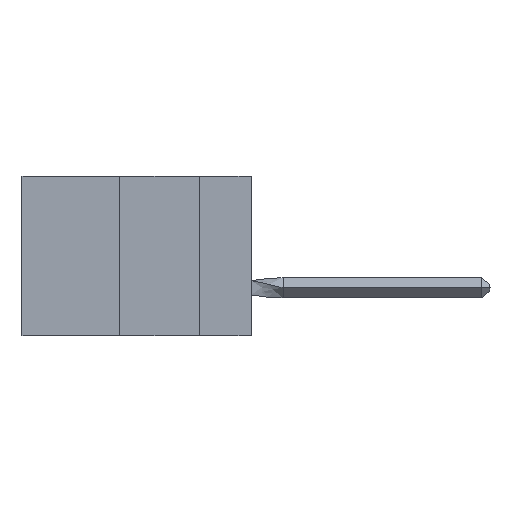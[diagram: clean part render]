
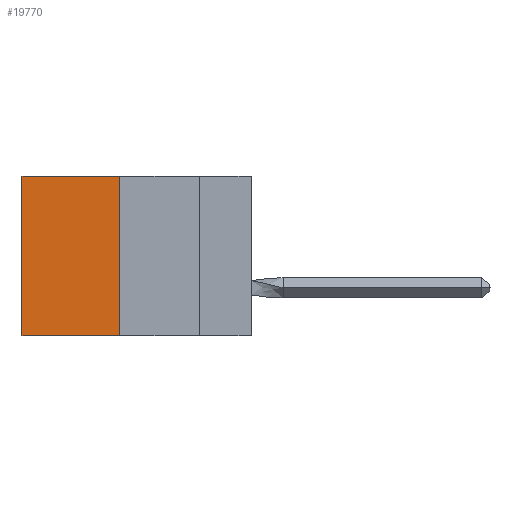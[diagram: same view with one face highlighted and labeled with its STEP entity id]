
A CAD part, left-side view. The second image highlights one B-rep face of the part: STEP entity #19770.
In plain terms, the highlighted planar face has unit normal (-1, 0, 0).
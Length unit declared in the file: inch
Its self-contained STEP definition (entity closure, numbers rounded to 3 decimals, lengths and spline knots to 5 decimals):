
#2408 = VERTEX_POINT ( 'NONE', #26722 ) ;
#3050 = VERTEX_POINT ( 'NONE', #18640 ) ;
#5060 = LINE ( 'NONE', #7306, #8090 ) ;
#5773 = DIRECTION ( 'NONE',  ( 1., 0., 0. ) ) ;
#5916 = CARTESIAN_POINT ( 'NONE',  ( 0.305, 0.413, -0.5 ) ) ;
#7297 = EDGE_CURVE ( 'NONE', #29053, #15346, #5060, .T. ) ;
#7306 = CARTESIAN_POINT ( 'NONE',  ( 0.305, 0.413, -0.5 ) ) ;
#8090 = VECTOR ( 'NONE', #20172, 39.37008 ) ;
#12396 = CARTESIAN_POINT ( 'NONE',  ( 0.305, 0.413, -0.5 ) ) ;
#14778 = VECTOR ( 'NONE', #28162, 39.37008 ) ;
#15084 = VECTOR ( 'NONE', #22329, 39.37008 ) ;
#15346 = VERTEX_POINT ( 'NONE', #33138 ) ;
#16229 = ORIENTED_EDGE ( 'NONE', *, *, #22057, .T. ) ;
#16317 = LINE ( 'NONE', #31427, #14778 ) ;
#16789 = EDGE_CURVE ( 'NONE', #3050, #15346, #28140, .T. ) ;
#17355 = LINE ( 'NONE', #12396, #22442 ) ;
#17820 = CARTESIAN_POINT ( 'NONE',  ( 0.305, 0.72, -0.5 ) ) ;
#18640 = CARTESIAN_POINT ( 'NONE',  ( 0.305, 0.72, 0. ) ) ;
#19770 = ADVANCED_FACE ( 'NONE', ( #37947 ), #38411, .F. ) ;
#19824 = EDGE_CURVE ( 'NONE', #2408, #29053, #17355, .T. ) ;
#20172 = DIRECTION ( 'NONE',  ( 0., 1., 0. ) ) ;
#22057 = EDGE_CURVE ( 'NONE', #2408, #3050, #16317, .T. ) ;
#22329 = DIRECTION ( 'NONE',  ( 0., 0., -1. ) ) ;
#22442 = VECTOR ( 'NONE', #28450, 39.37008 ) ;
#26722 = CARTESIAN_POINT ( 'NONE',  ( 0.305, 0.413, 0. ) ) ;
#28017 = AXIS2_PLACEMENT_3D ( 'NONE', #5916, #5773, #31833 ) ;
#28140 = LINE ( 'NONE', #17820, #15084 ) ;
#28162 = DIRECTION ( 'NONE',  ( 0., 1., 0. ) ) ;
#28173 = ORIENTED_EDGE ( 'NONE', *, *, #7297, .F. ) ;
#28450 = DIRECTION ( 'NONE',  ( 0., 0., -1. ) ) ;
#29053 = VERTEX_POINT ( 'NONE', #39777 ) ;
#31427 = CARTESIAN_POINT ( 'NONE',  ( 0.305, 0.413, 0. ) ) ;
#31610 = ORIENTED_EDGE ( 'NONE', *, *, #16789, .T. ) ;
#31833 = DIRECTION ( 'NONE',  ( 0., 0., -1. ) ) ;
#33138 = CARTESIAN_POINT ( 'NONE',  ( 0.305, 0.72, -0.5 ) ) ;
#35931 = ORIENTED_EDGE ( 'NONE', *, *, #19824, .F. ) ;
#37947 = FACE_OUTER_BOUND ( 'NONE', #40075, .T. ) ;
#38411 = PLANE ( 'NONE',  #28017 ) ;
#39777 = CARTESIAN_POINT ( 'NONE',  ( 0.305, 0.413, -0.5 ) ) ;
#40075 = EDGE_LOOP ( 'NONE', ( #31610, #28173, #35931, #16229 ) ) ;
